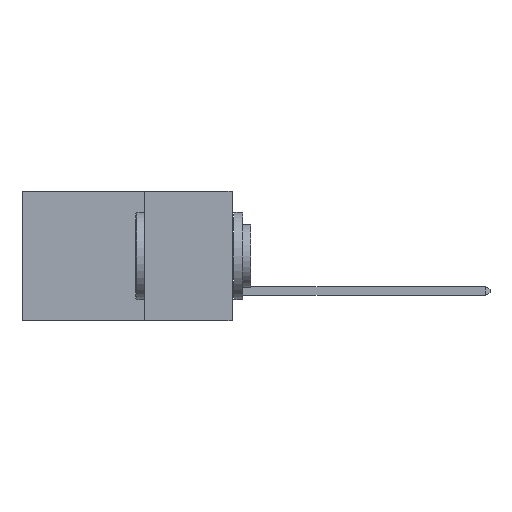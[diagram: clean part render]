
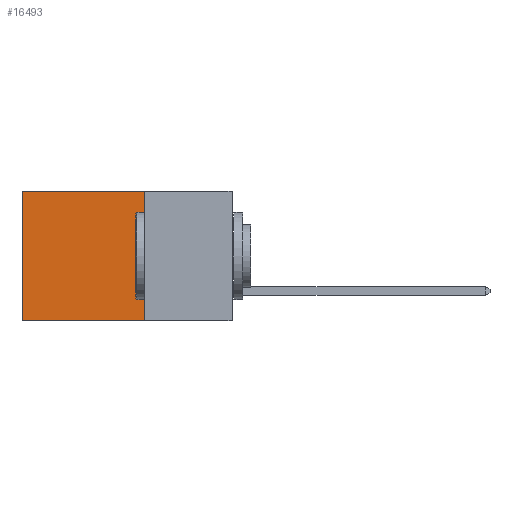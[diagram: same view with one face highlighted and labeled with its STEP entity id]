
A CAD part, left-side view. The second image highlights one B-rep face of the part: STEP entity #16493.
In plain terms, the highlighted planar face has unit normal (-1, 0, 0).
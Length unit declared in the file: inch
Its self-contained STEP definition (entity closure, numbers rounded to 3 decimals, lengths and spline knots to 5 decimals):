
#1194 = ORIENTED_EDGE ( 'NONE', *, *, #13134, .F. ) ;
#1422 = VECTOR ( 'NONE', #6844, 39.37008 ) ;
#1574 = FACE_OUTER_BOUND ( 'NONE', #5799, .T. ) ;
#1680 = CARTESIAN_POINT ( 'NONE',  ( 0.2875, 0.6, -0.37 ) ) ;
#3008 = DIRECTION ( 'NONE',  ( 0., 0., -1. ) ) ;
#3532 = ORIENTED_EDGE ( 'NONE', *, *, #11889, .F. ) ;
#4764 = CARTESIAN_POINT ( 'NONE',  ( 0.2875, 0.6, 0. ) ) ;
#5239 = CARTESIAN_POINT ( 'NONE',  ( 0.2875, 0.25, 0. ) ) ;
#5799 = EDGE_LOOP ( 'NONE', ( #18105, #3532, #1194, #15791 ) ) ;
#6060 = DIRECTION ( 'NONE',  ( 0., 1., 0. ) ) ;
#6844 = DIRECTION ( 'NONE',  ( 0., 0., -1. ) ) ;
#7320 = VERTEX_POINT ( 'NONE', #5239 ) ;
#8102 = VECTOR ( 'NONE', #12054, 39.37008 ) ;
#8362 = CARTESIAN_POINT ( 'NONE',  ( 0.2875, 0.25, -0.37 ) ) ;
#8710 = LINE ( 'NONE', #21695, #8102 ) ;
#9420 = LINE ( 'NONE', #19673, #23569 ) ;
#10357 = CARTESIAN_POINT ( 'NONE',  ( 0.2875, 0.25, 0. ) ) ;
#10549 = VERTEX_POINT ( 'NONE', #8362 ) ;
#11889 = EDGE_CURVE ( 'NONE', #10549, #15433, #8710, .T. ) ;
#12054 = DIRECTION ( 'NONE',  ( 0., 1., 0. ) ) ;
#12124 = LINE ( 'NONE', #4764, #1422 ) ;
#12249 = DIRECTION ( 'NONE',  ( 0., 0., -1. ) ) ;
#13134 = EDGE_CURVE ( 'NONE', #7320, #10549, #15127, .T. ) ;
#13332 = AXIS2_PLACEMENT_3D ( 'NONE', #18672, #14875, #3008 ) ;
#13642 = EDGE_CURVE ( 'NONE', #7320, #19966, #9420, .T. ) ;
#14875 = DIRECTION ( 'NONE',  ( 1., 0., 0. ) ) ;
#15127 = LINE ( 'NONE', #10357, #24764 ) ;
#15433 = VERTEX_POINT ( 'NONE', #1680 ) ;
#15791 = ORIENTED_EDGE ( 'NONE', *, *, #13642, .T. ) ;
#16493 = ADVANCED_FACE ( 'NONE', ( #1574 ), #24471, .F. ) ;
#18105 = ORIENTED_EDGE ( 'NONE', *, *, #21292, .T. ) ;
#18672 = CARTESIAN_POINT ( 'NONE',  ( 0.2875, 0.25, 0. ) ) ;
#19673 = CARTESIAN_POINT ( 'NONE',  ( 0.2875, 0.25, 0. ) ) ;
#19966 = VERTEX_POINT ( 'NONE', #22169 ) ;
#21292 = EDGE_CURVE ( 'NONE', #19966, #15433, #12124, .T. ) ;
#21695 = CARTESIAN_POINT ( 'NONE',  ( 0.2875, 0.25, -0.37 ) ) ;
#22169 = CARTESIAN_POINT ( 'NONE',  ( 0.2875, 0.6, 0. ) ) ;
#23569 = VECTOR ( 'NONE', #6060, 39.37008 ) ;
#24471 = PLANE ( 'NONE',  #13332 ) ;
#24764 = VECTOR ( 'NONE', #12249, 39.37008 ) ;
